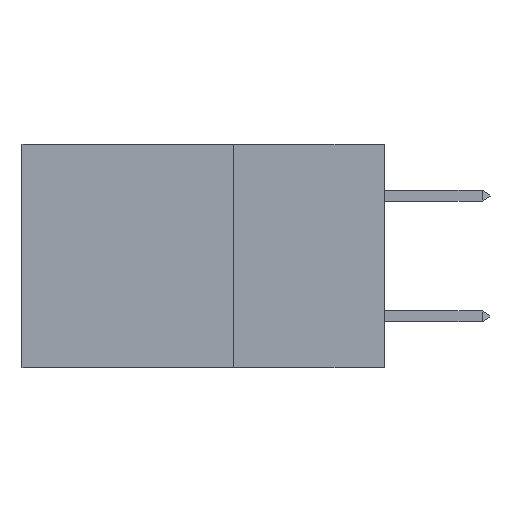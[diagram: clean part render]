
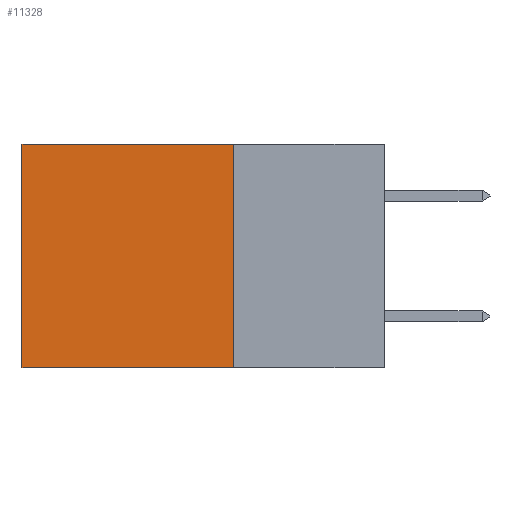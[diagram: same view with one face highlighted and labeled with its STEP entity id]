
A CAD part, left-side view. The second image highlights one B-rep face of the part: STEP entity #11328.
In plain terms, the highlighted planar face has unit normal (-1, 0, 0).
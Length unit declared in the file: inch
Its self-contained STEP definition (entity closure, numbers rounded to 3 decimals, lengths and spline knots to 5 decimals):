
#763 = EDGE_LOOP ( 'NONE', ( #12563, #7358, #6381, #13178 ) ) ;
#985 = DIRECTION ( 'NONE',  ( 1., 0., 0. ) ) ;
#1072 = CARTESIAN_POINT ( 'NONE',  ( 0.2875, 0.25, 0. ) ) ;
#1136 = DIRECTION ( 'NONE',  ( 0., 1., 0. ) ) ;
#1736 = VERTEX_POINT ( 'NONE', #7002 ) ;
#1881 = LINE ( 'NONE', #5946, #2733 ) ;
#2144 = LINE ( 'NONE', #8317, #12204 ) ;
#2733 = VECTOR ( 'NONE', #11122, 39.37008 ) ;
#2737 = CARTESIAN_POINT ( 'NONE',  ( 0.2875, 0.6, 0. ) ) ;
#3089 = CARTESIAN_POINT ( 'NONE',  ( 0.2875, 0.25, 0. ) ) ;
#3412 = DIRECTION ( 'NONE',  ( 0., 0., -1. ) ) ;
#3767 = DIRECTION ( 'NONE',  ( 0., 0., -1. ) ) ;
#4435 = CARTESIAN_POINT ( 'NONE',  ( 0.2875, 0.6, -0.37 ) ) ;
#5299 = EDGE_CURVE ( 'NONE', #1736, #5564, #1881, .T. ) ;
#5389 = VERTEX_POINT ( 'NONE', #7166 ) ;
#5564 = VERTEX_POINT ( 'NONE', #4435 ) ;
#5946 = CARTESIAN_POINT ( 'NONE',  ( 0.2875, 0.25, -0.37 ) ) ;
#6134 = EDGE_CURVE ( 'NONE', #9498, #1736, #7870, .T. ) ;
#6381 = ORIENTED_EDGE ( 'NONE', *, *, #6134, .F. ) ;
#6602 = AXIS2_PLACEMENT_3D ( 'NONE', #3089, #985, #3412 ) ;
#6727 = EDGE_CURVE ( 'NONE', #9498, #5389, #2144, .T. ) ;
#7002 = CARTESIAN_POINT ( 'NONE',  ( 0.2875, 0.25, -0.37 ) ) ;
#7166 = CARTESIAN_POINT ( 'NONE',  ( 0.2875, 0.6, 0. ) ) ;
#7358 = ORIENTED_EDGE ( 'NONE', *, *, #5299, .F. ) ;
#7870 = LINE ( 'NONE', #10024, #8768 ) ;
#7962 = VECTOR ( 'NONE', #3767, 39.37008 ) ;
#8317 = CARTESIAN_POINT ( 'NONE',  ( 0.2875, 0.25, 0. ) ) ;
#8768 = VECTOR ( 'NONE', #10951, 39.37008 ) ;
#9193 = FACE_OUTER_BOUND ( 'NONE', #763, .T. ) ;
#9498 = VERTEX_POINT ( 'NONE', #1072 ) ;
#10024 = CARTESIAN_POINT ( 'NONE',  ( 0.2875, 0.25, 0. ) ) ;
#10951 = DIRECTION ( 'NONE',  ( 0., 0., -1. ) ) ;
#11103 = LINE ( 'NONE', #2737, #7962 ) ;
#11122 = DIRECTION ( 'NONE',  ( 0., 1., 0. ) ) ;
#11328 = ADVANCED_FACE ( 'NONE', ( #9193 ), #13275, .F. ) ;
#12204 = VECTOR ( 'NONE', #1136, 39.37008 ) ;
#12563 = ORIENTED_EDGE ( 'NONE', *, *, #13012, .T. ) ;
#13012 = EDGE_CURVE ( 'NONE', #5389, #5564, #11103, .T. ) ;
#13178 = ORIENTED_EDGE ( 'NONE', *, *, #6727, .T. ) ;
#13275 = PLANE ( 'NONE',  #6602 ) ;
